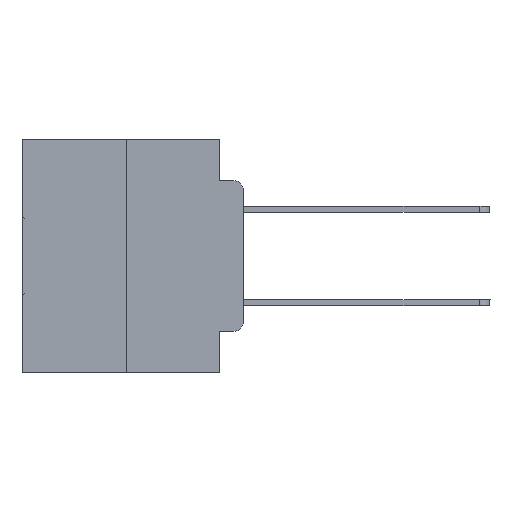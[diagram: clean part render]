
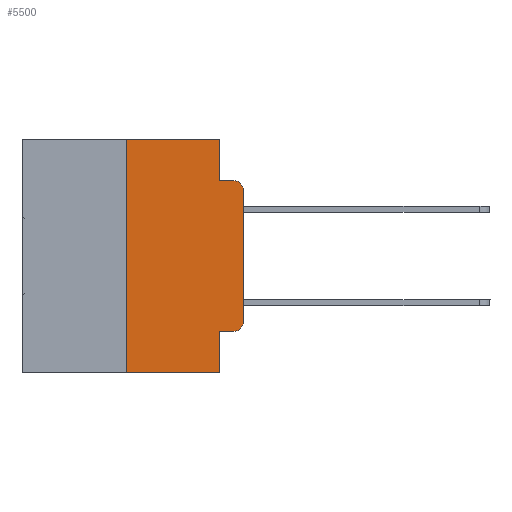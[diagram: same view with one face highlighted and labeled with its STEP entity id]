
A CAD part, left-side view. The second image highlights one B-rep face of the part: STEP entity #5500.
In plain terms, the highlighted planar face has unit normal (-1, 0, 0).
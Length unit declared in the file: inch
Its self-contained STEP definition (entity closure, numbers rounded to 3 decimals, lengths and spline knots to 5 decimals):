
#421 = EDGE_CURVE ( 'NONE', #1151, #22857, #25035, .T. ) ;
#476 = EDGE_LOOP ( 'NONE', ( #29406, #14930, #9231, #3328, #12248, #8219, #23201, #8121, #19367, #10274 ) ) ;
#608 = CIRCLE ( 'NONE', #1694, 0.02 ) ;
#1151 = VERTEX_POINT ( 'NONE', #14567 ) ;
#1218 = EDGE_CURVE ( 'NONE', #23851, #2525, #1546, .T. ) ;
#1546 = CIRCLE ( 'NONE', #9128, 0.02 ) ;
#1679 = VECTOR ( 'NONE', #25195, 39.37008 ) ;
#1694 = AXIS2_PLACEMENT_3D ( 'NONE', #2385, #21871, #21974 ) ;
#2385 = CARTESIAN_POINT ( 'NONE',  ( 0., 0.02, -0.3915 ) ) ;
#2525 = VERTEX_POINT ( 'NONE', #4335 ) ;
#2665 = CARTESIAN_POINT ( 'NONE',  ( 0., 0., -0.3915 ) ) ;
#2697 = CARTESIAN_POINT ( 'NONE',  ( 0., 0., 0. ) ) ;
#3328 = ORIENTED_EDGE ( 'NONE', *, *, #17713, .F. ) ;
#3361 = LINE ( 'NONE', #26007, #24333 ) ;
#3777 = DIRECTION ( 'NONE',  ( 0., -1., 0. ) ) ;
#4111 = LINE ( 'NONE', #15927, #17817 ) ;
#4335 = CARTESIAN_POINT ( 'NONE',  ( 0., 0.02, -0.0885 ) ) ;
#4558 = DIRECTION ( 'NONE',  ( 1., 0., 0. ) ) ;
#4857 = EDGE_CURVE ( 'NONE', #20529, #22689, #27687, .T. ) ;
#5500 = ADVANCED_FACE ( 'NONE', ( #10107 ), #9260, .F. ) ;
#7017 = CARTESIAN_POINT ( 'NONE',  ( 0., 0.473, 0. ) ) ;
#7070 = LINE ( 'NONE', #2697, #1679 ) ;
#7320 = LINE ( 'NONE', #29043, #21028 ) ;
#7931 = DIRECTION ( 'NONE',  ( 0., 0., -1. ) ) ;
#8022 = VERTEX_POINT ( 'NONE', #29926 ) ;
#8040 = CARTESIAN_POINT ( 'NONE',  ( 0., 0.02, -0.1085 ) ) ;
#8121 = ORIENTED_EDGE ( 'NONE', *, *, #421, .F. ) ;
#8198 = AXIS2_PLACEMENT_3D ( 'NONE', #7017, #4558, #9476 ) ;
#8219 = ORIENTED_EDGE ( 'NONE', *, *, #8335, .F. ) ;
#8335 = EDGE_CURVE ( 'NONE', #11544, #20529, #8826, .T. ) ;
#8826 = LINE ( 'NONE', #19238, #20983 ) ;
#8897 = LINE ( 'NONE', #30210, #27566 ) ;
#9128 = AXIS2_PLACEMENT_3D ( 'NONE', #8040, #10497, #7931 ) ;
#9231 = ORIENTED_EDGE ( 'NONE', *, *, #24229, .F. ) ;
#9260 = PLANE ( 'NONE',  #8198 ) ;
#9476 = DIRECTION ( 'NONE',  ( 0., 0., -1. ) ) ;
#9654 = DIRECTION ( 'NONE',  ( 0., 0., -1. ) ) ;
#10077 = CARTESIAN_POINT ( 'NONE',  ( 0., 0.051, 0. ) ) ;
#10107 = FACE_OUTER_BOUND ( 'NONE', #476, .T. ) ;
#10274 = ORIENTED_EDGE ( 'NONE', *, *, #10532, .T. ) ;
#10497 = DIRECTION ( 'NONE',  ( -1., 0., 0. ) ) ;
#10532 = EDGE_CURVE ( 'NONE', #8022, #17256, #608, .T. ) ;
#11222 = DIRECTION ( 'NONE',  ( 0., -1., 0. ) ) ;
#11544 = VERTEX_POINT ( 'NONE', #27804 ) ;
#12241 = CARTESIAN_POINT ( 'NONE',  ( 0., 0.473, 0. ) ) ;
#12248 = ORIENTED_EDGE ( 'NONE', *, *, #4857, .F. ) ;
#12305 = CARTESIAN_POINT ( 'NONE',  ( 0., 0.051, -0.0885 ) ) ;
#12852 = VECTOR ( 'NONE', #29499, 39.37008 ) ;
#13602 = EDGE_CURVE ( 'NONE', #11544, #22857, #8897, .T. ) ;
#14567 = CARTESIAN_POINT ( 'NONE',  ( 0., 0.051, -0.4115 ) ) ;
#14888 = EDGE_CURVE ( 'NONE', #17256, #23851, #7070, .T. ) ;
#14930 = ORIENTED_EDGE ( 'NONE', *, *, #1218, .T. ) ;
#15927 = CARTESIAN_POINT ( 'NONE',  ( 0., 0.051, -0.4115 ) ) ;
#16452 = CARTESIAN_POINT ( 'NONE',  ( 0., 0.051, 0. ) ) ;
#17256 = VERTEX_POINT ( 'NONE', #2665 ) ;
#17713 = EDGE_CURVE ( 'NONE', #22689, #27974, #7320, .T. ) ;
#17817 = VECTOR ( 'NONE', #3777, 39.37008 ) ;
#18187 = VECTOR ( 'NONE', #20552, 39.37008 ) ;
#19238 = CARTESIAN_POINT ( 'NONE',  ( 0., 0.25, 0. ) ) ;
#19367 = ORIENTED_EDGE ( 'NONE', *, *, #19617, .T. ) ;
#19617 = EDGE_CURVE ( 'NONE', #1151, #8022, #4111, .T. ) ;
#20350 = DIRECTION ( 'NONE',  ( 0., -1., 0. ) ) ;
#20529 = VERTEX_POINT ( 'NONE', #24373 ) ;
#20552 = DIRECTION ( 'NONE',  ( 0., 0., -1. ) ) ;
#20983 = VECTOR ( 'NONE', #28842, 39.37008 ) ;
#21028 = VECTOR ( 'NONE', #9654, 39.37008 ) ;
#21871 = DIRECTION ( 'NONE',  ( -1., 0., 0. ) ) ;
#21974 = DIRECTION ( 'NONE',  ( 0., 0., -1. ) ) ;
#22689 = VERTEX_POINT ( 'NONE', #16452 ) ;
#22857 = VERTEX_POINT ( 'NONE', #23816 ) ;
#23201 = ORIENTED_EDGE ( 'NONE', *, *, #13602, .T. ) ;
#23816 = CARTESIAN_POINT ( 'NONE',  ( 0., 0.051, -0.5 ) ) ;
#23851 = VERTEX_POINT ( 'NONE', #27500 ) ;
#24229 = EDGE_CURVE ( 'NONE', #27974, #2525, #3361, .T. ) ;
#24333 = VECTOR ( 'NONE', #11222, 39.37008 ) ;
#24373 = CARTESIAN_POINT ( 'NONE',  ( 0., 0.25, 0. ) ) ;
#25035 = LINE ( 'NONE', #10077, #18187 ) ;
#25195 = DIRECTION ( 'NONE',  ( 0., 0., 1. ) ) ;
#26007 = CARTESIAN_POINT ( 'NONE',  ( 0., 0.051, -0.0885 ) ) ;
#27500 = CARTESIAN_POINT ( 'NONE',  ( 0., 0., -0.1085 ) ) ;
#27566 = VECTOR ( 'NONE', #20350, 39.37008 ) ;
#27687 = LINE ( 'NONE', #12241, #12852 ) ;
#27804 = CARTESIAN_POINT ( 'NONE',  ( 0., 0.25, -0.5 ) ) ;
#27974 = VERTEX_POINT ( 'NONE', #12305 ) ;
#28842 = DIRECTION ( 'NONE',  ( 0., 0., 1. ) ) ;
#29043 = CARTESIAN_POINT ( 'NONE',  ( 0., 0.051, 0. ) ) ;
#29406 = ORIENTED_EDGE ( 'NONE', *, *, #14888, .T. ) ;
#29499 = DIRECTION ( 'NONE',  ( 0., -1., 0. ) ) ;
#29926 = CARTESIAN_POINT ( 'NONE',  ( 0., 0.02, -0.4115 ) ) ;
#30210 = CARTESIAN_POINT ( 'NONE',  ( 0., 0.473, -0.5 ) ) ;
